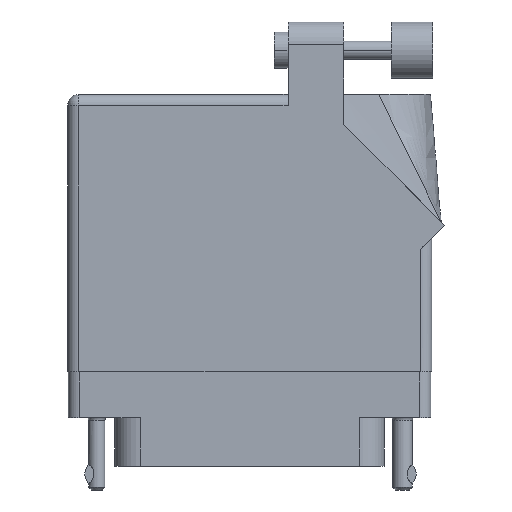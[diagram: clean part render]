
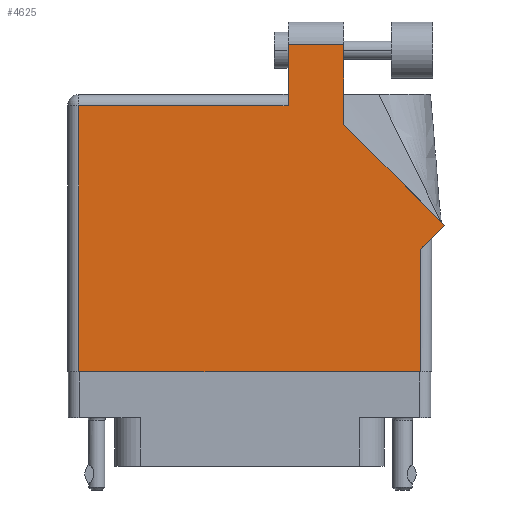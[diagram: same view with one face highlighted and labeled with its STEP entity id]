
A CAD part, front view. The second image highlights one B-rep face of the part: STEP entity #4625.
In plain terms, the highlighted face is planar.
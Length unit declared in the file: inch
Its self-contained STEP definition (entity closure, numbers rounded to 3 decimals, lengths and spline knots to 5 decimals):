
#266 = CARTESIAN_POINT ( 'NONE',  ( -1.005, 1.43, 0.455 ) ) ;
#335 = CARTESIAN_POINT ( 'NONE',  ( 0.943, 0.575, 0.455 ) ) ;
#1623 = ORIENTED_EDGE ( 'NONE', *, *, #40125, .T. ) ;
#1630 = LINE ( 'NONE', #31781, #3405 ) ;
#1844 = ORIENTED_EDGE ( 'NONE', *, *, #9160, .T. ) ;
#1883 = VECTOR ( 'NONE', #22599, 39.37008 ) ;
#1939 = DIRECTION ( 'NONE',  ( 0., -1., 0. ) ) ;
#2242 = VERTEX_POINT ( 'NONE', #6066 ) ;
#3245 = CARTESIAN_POINT ( 'NONE',  ( 1.07571, 0.70771, 0.455 ) ) ;
#3405 = VECTOR ( 'NONE', #12843, 39.37008 ) ;
#3626 = CARTESIAN_POINT ( 'NONE',  ( 0.519, 1.705, 0.455 ) ) ;
#4625 = ADVANCED_FACE ( 'NONE', ( #9331 ), #30984, .F. ) ;
#4814 = ORIENTED_EDGE ( 'NONE', *, *, #16959, .T. ) ;
#5406 = CARTESIAN_POINT ( 'NONE',  ( 0.519, 1.26442, 0.455 ) ) ;
#5524 = ORIENTED_EDGE ( 'NONE', *, *, #12788, .T. ) ;
#5791 = VECTOR ( 'NONE', #43232, 39.37008 ) ;
#6066 = CARTESIAN_POINT ( 'NONE',  ( 1.07571, 0.70771, 0.455 ) ) ;
#6149 = VERTEX_POINT ( 'NONE', #3626 ) ;
#6922 = CARTESIAN_POINT ( 'NONE',  ( 1.005, 0.637, 0.455 ) ) ;
#7251 = DIRECTION ( 'NONE',  ( 0.707, 0.707, 0. ) ) ;
#8048 = LINE ( 'NONE', #5406, #31817 ) ;
#8226 = DIRECTION ( 'NONE',  ( -1., 0., 0. ) ) ;
#8669 = DIRECTION ( 'NONE',  ( 1., 0., 0. ) ) ;
#9160 = EDGE_CURVE ( 'NONE', #22877, #38833, #31485, .T. ) ;
#9331 = FACE_OUTER_BOUND ( 'NONE', #19808, .T. ) ;
#10133 = AXIS2_PLACEMENT_3D ( 'NONE', #266, #30653, #8226 ) ;
#10666 = LINE ( 'NONE', #20114, #46971 ) ;
#11925 = CARTESIAN_POINT ( 'NONE',  ( -0.943, -0.1, 0.455 ) ) ;
#11990 = LINE ( 'NONE', #14908, #1883 ) ;
#12013 = DIRECTION ( 'NONE',  ( 0., -1., 0. ) ) ;
#12788 = EDGE_CURVE ( 'NONE', #2242, #39841, #34735, .T. ) ;
#12843 = DIRECTION ( 'NONE',  ( -1., 0., 0. ) ) ;
#14908 = CARTESIAN_POINT ( 'NONE',  ( -1.005, 1.368, 0.455 ) ) ;
#16639 = DIRECTION ( 'NONE',  ( 0., 1., 0. ) ) ;
#16959 = EDGE_CURVE ( 'NONE', #23988, #22877, #11990, .T. ) ;
#18317 = DIRECTION ( 'NONE',  ( -0.707, 0.707, 0. ) ) ;
#19306 = EDGE_CURVE ( 'NONE', #38833, #19757, #10666, .T. ) ;
#19757 = VERTEX_POINT ( 'NONE', #30523 ) ;
#19797 = CARTESIAN_POINT ( 'NONE',  ( -0.943, -0.1, 0.455 ) ) ;
#19808 = EDGE_LOOP ( 'NONE', ( #48291, #42881, #34497, #4814, #1844, #45907, #1623, #39512, #5524 ) ) ;
#20114 = CARTESIAN_POINT ( 'NONE',  ( -1.005, -0.1, 0.455 ) ) ;
#20353 = CARTESIAN_POINT ( 'NONE',  ( 0.212, 1.705, 0.455 ) ) ;
#22599 = DIRECTION ( 'NONE',  ( -1., 0., 0. ) ) ;
#22841 = VERTEX_POINT ( 'NONE', #20353 ) ;
#22877 = VERTEX_POINT ( 'NONE', #35795 ) ;
#23620 = CARTESIAN_POINT ( 'NONE',  ( 0.943, 0.637, 0.455 ) ) ;
#23860 = LINE ( 'NONE', #31994, #26221 ) ;
#23988 = VERTEX_POINT ( 'NONE', #36529 ) ;
#25538 = VECTOR ( 'NONE', #12013, 39.37008 ) ;
#26221 = VECTOR ( 'NONE', #1939, 39.37008 ) ;
#29372 = VERTEX_POINT ( 'NONE', #335 ) ;
#30361 = VECTOR ( 'NONE', #7251, 39.37008 ) ;
#30523 = CARTESIAN_POINT ( 'NONE',  ( 0.943, -0.1, 0.455 ) ) ;
#30653 = DIRECTION ( 'NONE',  ( 0., 0., -1. ) ) ;
#30984 = PLANE ( 'NONE',  #10133 ) ;
#31485 = LINE ( 'NONE', #19797, #25538 ) ;
#31488 = EDGE_CURVE ( 'NONE', #39841, #6149, #8048, .T. ) ;
#31781 = CARTESIAN_POINT ( 'NONE',  ( 0.212, 1.705, 0.455 ) ) ;
#31817 = VECTOR ( 'NONE', #16639, 39.37008 ) ;
#31994 = CARTESIAN_POINT ( 'NONE',  ( 0.212, 1.43, 0.455 ) ) ;
#34497 = ORIENTED_EDGE ( 'NONE', *, *, #44389, .T. ) ;
#34735 = LINE ( 'NONE', #3245, #40121 ) ;
#35107 = LINE ( 'NONE', #6922, #30361 ) ;
#35795 = CARTESIAN_POINT ( 'NONE',  ( -0.943, 1.368, 0.455 ) ) ;
#36085 = LINE ( 'NONE', #23620, #5791 ) ;
#36529 = CARTESIAN_POINT ( 'NONE',  ( 0.212, 1.368, 0.455 ) ) ;
#38833 = VERTEX_POINT ( 'NONE', #11925 ) ;
#39375 = EDGE_CURVE ( 'NONE', #6149, #22841, #1630, .T. ) ;
#39512 = ORIENTED_EDGE ( 'NONE', *, *, #46391, .T. ) ;
#39841 = VERTEX_POINT ( 'NONE', #41641 ) ;
#40121 = VECTOR ( 'NONE', #18317, 39.37008 ) ;
#40125 = EDGE_CURVE ( 'NONE', #19757, #29372, #36085, .T. ) ;
#41641 = CARTESIAN_POINT ( 'NONE',  ( 0.519, 1.26442, 0.455 ) ) ;
#42881 = ORIENTED_EDGE ( 'NONE', *, *, #39375, .T. ) ;
#43232 = DIRECTION ( 'NONE',  ( 0., 1., 0. ) ) ;
#44389 = EDGE_CURVE ( 'NONE', #22841, #23988, #23860, .T. ) ;
#45907 = ORIENTED_EDGE ( 'NONE', *, *, #19306, .T. ) ;
#46391 = EDGE_CURVE ( 'NONE', #29372, #2242, #35107, .T. ) ;
#46971 = VECTOR ( 'NONE', #8669, 39.37008 ) ;
#48291 = ORIENTED_EDGE ( 'NONE', *, *, #31488, .T. ) ;
